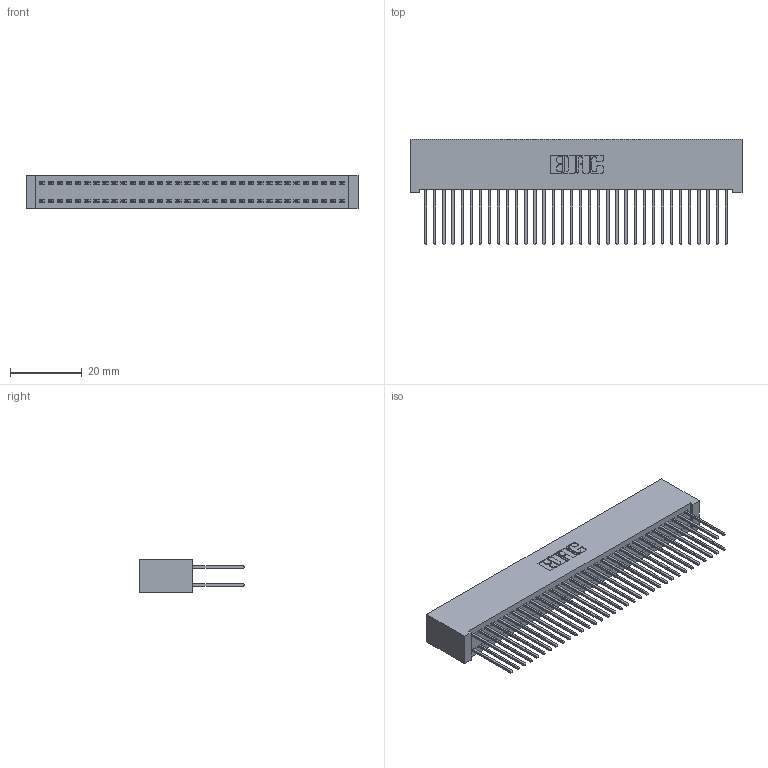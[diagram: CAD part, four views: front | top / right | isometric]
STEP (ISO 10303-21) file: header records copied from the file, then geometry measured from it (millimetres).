
FILE_DESCRIPTION (( 'STEP AP203' ), '1' );
FILE_NAME ('392-068-540-201.STEP', '2018-08-17T22:47:34', ( '' ), ( '' ), 'SwSTEP 2.0', 'SolidWorks 2016', '' );
FILE_SCHEMA (( 'CONFIG_CONTROL_DESIGN' ));
Length unit declared in the file: inch
Products named in the file (3): 342 Part_Lugless; 345-292-001_345-293-140; 392-068-540-201
Assembly tree (69 placements, depth 2):
  392-068-540-201
    342 Part_Lugless
    345-292-001_345-293-140  x68
Bounding box: 92.61 x 29.47 x 9.4 mm (x, y, z)
Volume: 8980.3 mm3; surface area: 16012.8 mm2
Topology: 69 solids, 69 shells, 3638 faces, 10815 edges, 7118 vertices
Faces by surface type: plane 2510, cylinder 1128
Entity records: 22517 total; most frequent: CARTESIAN_POINT 3738, ORIENTED_EDGE 3674, DIRECTION 3201, EDGE_CURVE 1837, VECTOR 1717, LINE 1717, VERTEX_POINT 1222, AXIS2_PLACEMENT_3D 742
